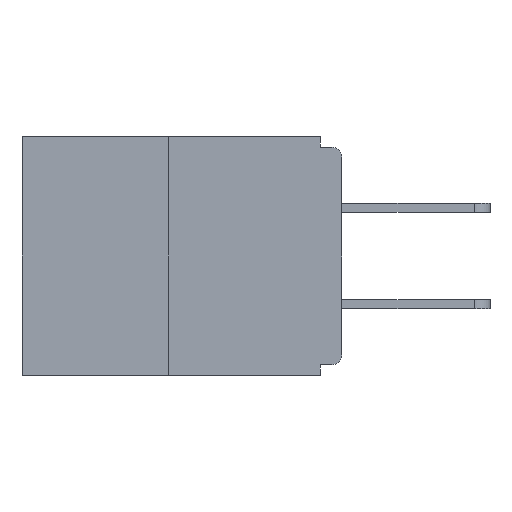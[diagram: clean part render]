
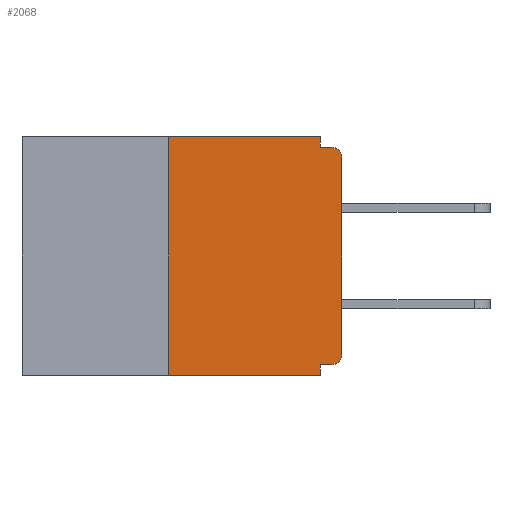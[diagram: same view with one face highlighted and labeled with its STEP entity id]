
A CAD part, left-side view. The second image highlights one B-rep face of the part: STEP entity #2068.
In plain terms, the highlighted planar face has unit normal (-1, 0, 0).
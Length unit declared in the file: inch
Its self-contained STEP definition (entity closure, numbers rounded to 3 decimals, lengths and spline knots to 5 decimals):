
#301 = LINE ( 'NONE', #1524, #6266 ) ;
#980 = DIRECTION ( 'NONE',  ( -1., 0., 0. ) ) ;
#1270 = EDGE_CURVE ( 'NONE', #17844, #11417, #8042, .T. ) ;
#1524 = CARTESIAN_POINT ( 'NONE',  ( 0., 0., -0.015 ) ) ;
#1528 = CARTESIAN_POINT ( 'NONE',  ( 0., 0., -0.328 ) ) ;
#1570 = EDGE_CURVE ( 'NONE', #17844, #16993, #8015, .T. ) ;
#1620 = DIRECTION ( 'NONE',  ( 0., 1., 0. ) ) ;
#1683 = DIRECTION ( 'NONE',  ( 0., 0., 1. ) ) ;
#2068 = ADVANCED_FACE ( 'NONE', ( #11244 ), #18940, .F. ) ;
#2086 = ORIENTED_EDGE ( 'NONE', *, *, #24029, .F. ) ;
#2852 = CARTESIAN_POINT ( 'NONE',  ( 0., 0.015, -0.015 ) ) ;
#3404 = VECTOR ( 'NONE', #13018, 39.37008 ) ;
#3478 = AXIS2_PLACEMENT_3D ( 'NONE', #19580, #8012, #15839 ) ;
#3795 = DIRECTION ( 'NONE',  ( 1., 0., 0. ) ) ;
#4730 = DIRECTION ( 'NONE',  ( 0., 0., 1. ) ) ;
#4885 = ORIENTED_EDGE ( 'NONE', *, *, #19978, .T. ) ;
#5116 = AXIS2_PLACEMENT_3D ( 'NONE', #7543, #3795, #9523 ) ;
#6071 = VERTEX_POINT ( 'NONE', #22746 ) ;
#6266 = VECTOR ( 'NONE', #24638, 39.37008 ) ;
#6606 = VECTOR ( 'NONE', #17956, 39.37008 ) ;
#7167 = EDGE_CURVE ( 'NONE', #16993, #19401, #17235, .T. ) ;
#7240 = LINE ( 'NONE', #1528, #12859 ) ;
#7543 = CARTESIAN_POINT ( 'NONE',  ( 0., 0.46, 0. ) ) ;
#7715 = CARTESIAN_POINT ( 'NONE',  ( 0., 0.031, 0. ) ) ;
#8003 = VERTEX_POINT ( 'NONE', #9476 ) ;
#8012 = DIRECTION ( 'NONE',  ( -1., 0., 0. ) ) ;
#8015 = LINE ( 'NONE', #9214, #14254 ) ;
#8042 = LINE ( 'NONE', #16026, #15788 ) ;
#8266 = ORIENTED_EDGE ( 'NONE', *, *, #7167, .F. ) ;
#8365 = ORIENTED_EDGE ( 'NONE', *, *, #13265, .F. ) ;
#8411 = CARTESIAN_POINT ( 'NONE',  ( 0., 0.015, -0.328 ) ) ;
#8672 = LINE ( 'NONE', #20062, #6606 ) ;
#9214 = CARTESIAN_POINT ( 'NONE',  ( 0., 0.25, 0. ) ) ;
#9476 = CARTESIAN_POINT ( 'NONE',  ( 0., 0.031, -0.328 ) ) ;
#9523 = DIRECTION ( 'NONE',  ( 0., 0., -1. ) ) ;
#10295 = VERTEX_POINT ( 'NONE', #21903 ) ;
#11090 = EDGE_CURVE ( 'NONE', #19401, #22103, #23352, .T. ) ;
#11244 = FACE_OUTER_BOUND ( 'NONE', #19464, .T. ) ;
#11417 = VERTEX_POINT ( 'NONE', #24502 ) ;
#11663 = EDGE_CURVE ( 'NONE', #23063, #8003, #7240, .T. ) ;
#12084 = CARTESIAN_POINT ( 'NONE',  ( 0., 0.031, -0.015 ) ) ;
#12151 = DIRECTION ( 'NONE',  ( 0., -1., 0. ) ) ;
#12161 = CARTESIAN_POINT ( 'NONE',  ( 0., 0., 0. ) ) ;
#12381 = CARTESIAN_POINT ( 'NONE',  ( 0., 0.25, 0. ) ) ;
#12663 = ORIENTED_EDGE ( 'NONE', *, *, #11663, .F. ) ;
#12859 = VECTOR ( 'NONE', #1620, 39.37008 ) ;
#13018 = DIRECTION ( 'NONE',  ( 0., 0., -1. ) ) ;
#13265 = EDGE_CURVE ( 'NONE', #22103, #13524, #301, .T. ) ;
#13524 = VERTEX_POINT ( 'NONE', #2852 ) ;
#13633 = VECTOR ( 'NONE', #24486, 39.37008 ) ;
#14027 = CARTESIAN_POINT ( 'NONE',  ( 0., 0.015, -0.03 ) ) ;
#14171 = CIRCLE ( 'NONE', #3478, 0.015 ) ;
#14254 = VECTOR ( 'NONE', #1683, 39.37008 ) ;
#14611 = EDGE_CURVE ( 'NONE', #10295, #13524, #15193, .T. ) ;
#15193 = CIRCLE ( 'NONE', #24458, 0.015 ) ;
#15788 = VECTOR ( 'NONE', #12151, 39.37008 ) ;
#15839 = DIRECTION ( 'NONE',  ( 0., 0., -1. ) ) ;
#16026 = CARTESIAN_POINT ( 'NONE',  ( 0., 0.46, -0.343 ) ) ;
#16200 = ORIENTED_EDGE ( 'NONE', *, *, #1570, .F. ) ;
#16346 = ORIENTED_EDGE ( 'NONE', *, *, #14611, .T. ) ;
#16993 = VERTEX_POINT ( 'NONE', #12381 ) ;
#17235 = LINE ( 'NONE', #18496, #13633 ) ;
#17722 = EDGE_CURVE ( 'NONE', #23063, #6071, #14171, .T. ) ;
#17844 = VERTEX_POINT ( 'NONE', #23553 ) ;
#17956 = DIRECTION ( 'NONE',  ( 0., 0., -1. ) ) ;
#18496 = CARTESIAN_POINT ( 'NONE',  ( 0., 0.46, 0. ) ) ;
#18940 = PLANE ( 'NONE',  #5116 ) ;
#19401 = VERTEX_POINT ( 'NONE', #23074 ) ;
#19464 = EDGE_LOOP ( 'NONE', ( #8266, #16200, #24059, #2086, #12663, #23911, #4885, #16346, #8365, #23093 ) ) ;
#19580 = CARTESIAN_POINT ( 'NONE',  ( 0., 0.015, -0.313 ) ) ;
#19739 = VECTOR ( 'NONE', #4730, 39.37008 ) ;
#19978 = EDGE_CURVE ( 'NONE', #6071, #10295, #23855, .T. ) ;
#20062 = CARTESIAN_POINT ( 'NONE',  ( 0., 0.031, -0.343 ) ) ;
#21777 = DIRECTION ( 'NONE',  ( 0., 0., -1. ) ) ;
#21903 = CARTESIAN_POINT ( 'NONE',  ( 0., 0., -0.03 ) ) ;
#22103 = VERTEX_POINT ( 'NONE', #12084 ) ;
#22746 = CARTESIAN_POINT ( 'NONE',  ( 0., 0., -0.313 ) ) ;
#23063 = VERTEX_POINT ( 'NONE', #8411 ) ;
#23074 = CARTESIAN_POINT ( 'NONE',  ( 0., 0.031, 0. ) ) ;
#23093 = ORIENTED_EDGE ( 'NONE', *, *, #11090, .F. ) ;
#23352 = LINE ( 'NONE', #7715, #3404 ) ;
#23553 = CARTESIAN_POINT ( 'NONE',  ( 0., 0.25, -0.343 ) ) ;
#23855 = LINE ( 'NONE', #12161, #19739 ) ;
#23911 = ORIENTED_EDGE ( 'NONE', *, *, #17722, .T. ) ;
#24029 = EDGE_CURVE ( 'NONE', #8003, #11417, #8672, .T. ) ;
#24059 = ORIENTED_EDGE ( 'NONE', *, *, #1270, .T. ) ;
#24458 = AXIS2_PLACEMENT_3D ( 'NONE', #14027, #980, #21777 ) ;
#24486 = DIRECTION ( 'NONE',  ( 0., -1., 0. ) ) ;
#24502 = CARTESIAN_POINT ( 'NONE',  ( 0., 0.031, -0.343 ) ) ;
#24638 = DIRECTION ( 'NONE',  ( 0., -1., 0. ) ) ;
